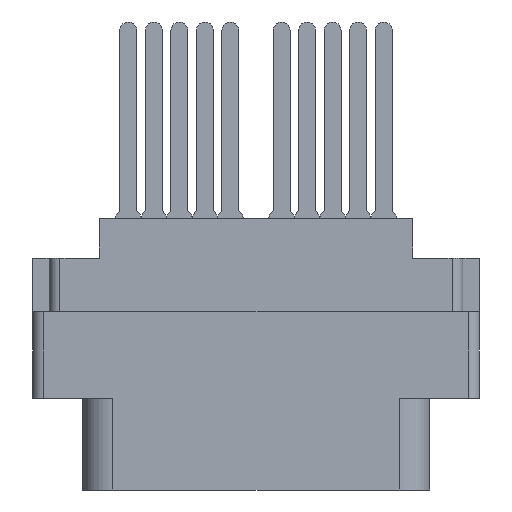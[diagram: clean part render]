
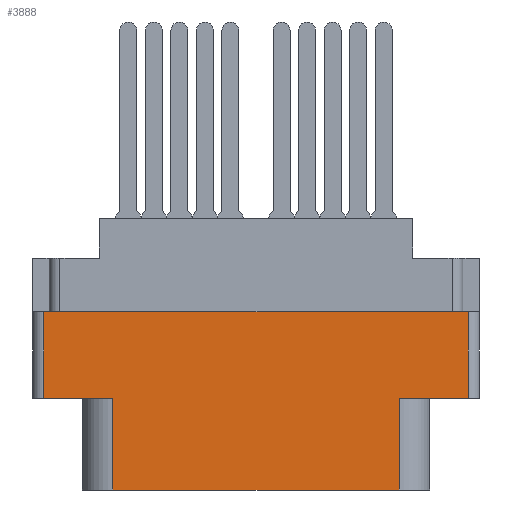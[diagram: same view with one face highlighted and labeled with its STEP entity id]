
A CAD part, front view. The second image highlights one B-rep face of the part: STEP entity #3888.
In plain terms, the highlighted planar face has unit normal (0, -1, 0).
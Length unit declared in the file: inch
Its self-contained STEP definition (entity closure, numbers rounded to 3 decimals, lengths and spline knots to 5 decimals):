
#187 = VERTEX_POINT ( 'NONE', #4015 ) ;
#1350 = DIRECTION ( 'NONE',  ( 0., -1., 0. ) ) ;
#1502 = VECTOR ( 'NONE', #25056, 39.37008 ) ;
#1508 = ORIENTED_EDGE ( 'NONE', *, *, #28106, .F. ) ;
#2144 = LINE ( 'NONE', #9423, #26378 ) ;
#2918 = VECTOR ( 'NONE', #23080, 39.37008 ) ;
#3716 = CARTESIAN_POINT ( 'NONE',  ( -0.624, -0.343, -0.529 ) ) ;
#3888 = ADVANCED_FACE ( 'NONE', ( #19666 ), #16285, .T. ) ;
#4015 = CARTESIAN_POINT ( 'NONE',  ( -0.624, -0.343, -0.274 ) ) ;
#4837 = EDGE_CURVE ( 'NONE', #187, #10712, #15200, .T. ) ;
#5133 = CARTESIAN_POINT ( 'NONE',  ( 0., -0.343, -0.529 ) ) ;
#5362 = ORIENTED_EDGE ( 'NONE', *, *, #4837, .F. ) ;
#5695 = LINE ( 'NONE', #14378, #2918 ) ;
#5860 = CARTESIAN_POINT ( 'NONE',  ( 0., -0.343, -0.274 ) ) ;
#6360 = EDGE_CURVE ( 'NONE', #26510, #21894, #12054, .T. ) ;
#6443 = DIRECTION ( 'NONE',  ( 1., 0., 0. ) ) ;
#6940 = ORIENTED_EDGE ( 'NONE', *, *, #7602, .T. ) ;
#7030 = CARTESIAN_POINT ( 'NONE',  ( -0.42052, -0.343, -0.529 ) ) ;
#7417 = DIRECTION ( 'NONE',  ( 1., 0., 0. ) ) ;
#7602 = EDGE_CURVE ( 'NONE', #27375, #10712, #27678, .T. ) ;
#8169 = DIRECTION ( 'NONE',  ( 1., 0., 0. ) ) ;
#9423 = CARTESIAN_POINT ( 'NONE',  ( -0.656, -0.343, -0.798 ) ) ;
#9471 = ORIENTED_EDGE ( 'NONE', *, *, #25548, .T. ) ;
#9678 = CARTESIAN_POINT ( 'NONE',  ( 0.42052, -0.343, -0.529 ) ) ;
#10068 = DIRECTION ( 'NONE',  ( 0., 0., 1. ) ) ;
#10285 = VECTOR ( 'NONE', #16850, 39.37008 ) ;
#10489 = CARTESIAN_POINT ( 'NONE',  ( 0., -0.343, -0.529 ) ) ;
#10712 = VERTEX_POINT ( 'NONE', #19073 ) ;
#11007 = EDGE_CURVE ( 'NONE', #14577, #15109, #11175, .T. ) ;
#11175 = LINE ( 'NONE', #9678, #27892 ) ;
#11917 = DIRECTION ( 'NONE',  ( -1., 0., 0. ) ) ;
#12054 = LINE ( 'NONE', #10489, #13431 ) ;
#13431 = VECTOR ( 'NONE', #8169, 39.37008 ) ;
#13509 = VECTOR ( 'NONE', #6443, 39.37008 ) ;
#14378 = CARTESIAN_POINT ( 'NONE',  ( -0.42052, -0.343, -0.798 ) ) ;
#14577 = VERTEX_POINT ( 'NONE', #23659 ) ;
#15109 = VERTEX_POINT ( 'NONE', #21812 ) ;
#15200 = LINE ( 'NONE', #5860, #13509 ) ;
#15836 = ORIENTED_EDGE ( 'NONE', *, *, #22139, .T. ) ;
#16285 = PLANE ( 'NONE',  #16360 ) ;
#16360 = AXIS2_PLACEMENT_3D ( 'NONE', #18553, #1350, #16648 ) ;
#16648 = DIRECTION ( 'NONE',  ( 0., 0., -1. ) ) ;
#16850 = DIRECTION ( 'NONE',  ( 0., 0., 1. ) ) ;
#18553 = CARTESIAN_POINT ( 'NONE',  ( -0.656, -0.343, -0.798 ) ) ;
#18939 = LINE ( 'NONE', #22603, #1502 ) ;
#19007 = VECTOR ( 'NONE', #11917, 39.37008 ) ;
#19073 = CARTESIAN_POINT ( 'NONE',  ( 0.624, -0.343, -0.274 ) ) ;
#19237 = CARTESIAN_POINT ( 'NONE',  ( 0.624, -0.343, -0.798 ) ) ;
#19273 = ORIENTED_EDGE ( 'NONE', *, *, #11007, .T. ) ;
#19314 = EDGE_LOOP ( 'NONE', ( #5362, #9471, #25846, #15836, #22887, #19273, #1508, #6940 ) ) ;
#19666 = FACE_OUTER_BOUND ( 'NONE', #19314, .T. ) ;
#21402 = CARTESIAN_POINT ( 'NONE',  ( -0.42052, -0.343, -0.798 ) ) ;
#21812 = CARTESIAN_POINT ( 'NONE',  ( 0.42052, -0.343, -0.529 ) ) ;
#21894 = VERTEX_POINT ( 'NONE', #7030 ) ;
#22139 = EDGE_CURVE ( 'NONE', #21894, #27793, #5695, .T. ) ;
#22603 = CARTESIAN_POINT ( 'NONE',  ( -0.624, -0.343, -0.798 ) ) ;
#22887 = ORIENTED_EDGE ( 'NONE', *, *, #26323, .T. ) ;
#23080 = DIRECTION ( 'NONE',  ( 0., 0., -1. ) ) ;
#23659 = CARTESIAN_POINT ( 'NONE',  ( 0.42052, -0.343, -0.798 ) ) ;
#25056 = DIRECTION ( 'NONE',  ( 0., 0., -1. ) ) ;
#25548 = EDGE_CURVE ( 'NONE', #187, #26510, #18939, .T. ) ;
#25846 = ORIENTED_EDGE ( 'NONE', *, *, #6360, .T. ) ;
#26323 = EDGE_CURVE ( 'NONE', #27793, #14577, #2144, .T. ) ;
#26378 = VECTOR ( 'NONE', #7417, 39.37008 ) ;
#26510 = VERTEX_POINT ( 'NONE', #3716 ) ;
#26615 = CARTESIAN_POINT ( 'NONE',  ( 0.624, -0.343, -0.529 ) ) ;
#26835 = LINE ( 'NONE', #5133, #19007 ) ;
#27375 = VERTEX_POINT ( 'NONE', #26615 ) ;
#27678 = LINE ( 'NONE', #19237, #10285 ) ;
#27793 = VERTEX_POINT ( 'NONE', #21402 ) ;
#27892 = VECTOR ( 'NONE', #10068, 39.37008 ) ;
#28106 = EDGE_CURVE ( 'NONE', #27375, #15109, #26835, .T. ) ;
